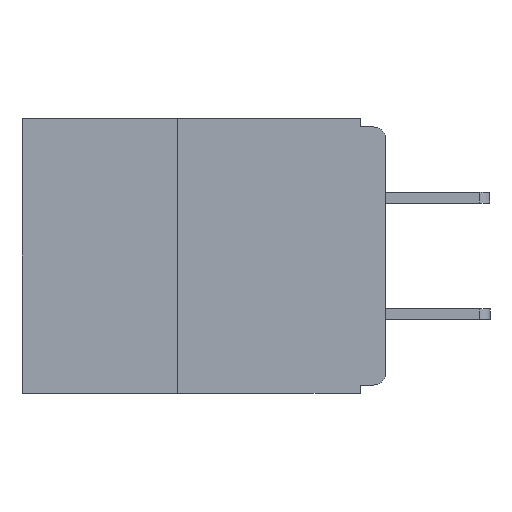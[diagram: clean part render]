
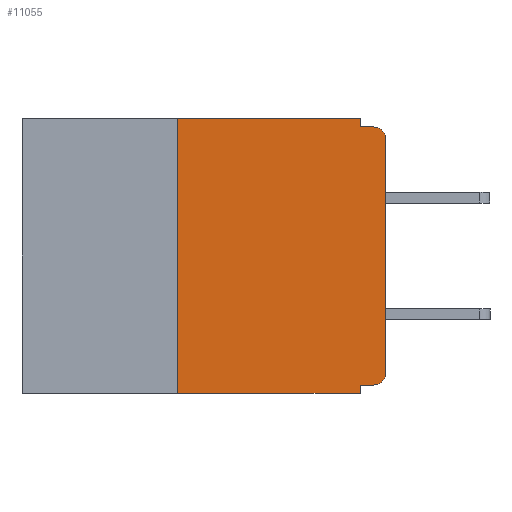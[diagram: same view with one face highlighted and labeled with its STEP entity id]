
A CAD part, left-side view. The second image highlights one B-rep face of the part: STEP entity #11055.
In plain terms, the highlighted planar face has unit normal (-1, 0, 0).
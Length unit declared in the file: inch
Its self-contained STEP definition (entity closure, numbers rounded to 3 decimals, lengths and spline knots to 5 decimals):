
#9 = VECTOR ( 'NONE', #11771, 39.37008 ) ;
#267 = DIRECTION ( 'NONE',  ( 0., 1., 0. ) ) ;
#414 = DIRECTION ( 'NONE',  ( 0., 0., -1. ) ) ;
#440 = ORIENTED_EDGE ( 'NONE', *, *, #5736, .T. ) ;
#484 = AXIS2_PLACEMENT_3D ( 'NONE', #6785, #6767, #6724 ) ;
#1037 = VECTOR ( 'NONE', #15498, 39.37008 ) ;
#1721 = EDGE_CURVE ( 'NONE', #16493, #3948, #3921, .T. ) ;
#1986 = FACE_OUTER_BOUND ( 'NONE', #13080, .T. ) ;
#2492 = EDGE_CURVE ( 'NONE', #4934, #12769, #3906, .T. ) ;
#2823 = LINE ( 'NONE', #11462, #10269 ) ;
#3153 = DIRECTION ( 'NONE',  ( 0., 0., 1. ) ) ;
#3399 = VERTEX_POINT ( 'NONE', #6399 ) ;
#3489 = CARTESIAN_POINT ( 'NONE',  ( 0., 0.031, 0. ) ) ;
#3809 = CARTESIAN_POINT ( 'NONE',  ( 0., 0., -0.32 ) ) ;
#3897 = CARTESIAN_POINT ( 'NONE',  ( 0., 0.031, -0.01 ) ) ;
#3906 = LINE ( 'NONE', #8156, #9 ) ;
#3921 = LINE ( 'NONE', #3809, #10933 ) ;
#3948 = VERTEX_POINT ( 'NONE', #5314 ) ;
#4382 = CARTESIAN_POINT ( 'NONE',  ( 0., 0., -0.305 ) ) ;
#4439 = CIRCLE ( 'NONE', #484, 0.015 ) ;
#4491 = DIRECTION ( 'NONE',  ( 0., -1., 0. ) ) ;
#4507 = CARTESIAN_POINT ( 'NONE',  ( 0., 0., -0.01 ) ) ;
#4882 = CARTESIAN_POINT ( 'NONE',  ( 0., 0.015, -0.01 ) ) ;
#4893 = VERTEX_POINT ( 'NONE', #4382 ) ;
#4934 = VERTEX_POINT ( 'NONE', #3489 ) ;
#5068 = LINE ( 'NONE', #12923, #12926 ) ;
#5070 = LINE ( 'NONE', #6970, #8335 ) ;
#5104 = VECTOR ( 'NONE', #5201, 39.37008 ) ;
#5185 = CARTESIAN_POINT ( 'NONE',  ( 0., 0.031, -0.33 ) ) ;
#5201 = DIRECTION ( 'NONE',  ( 0., 0., -1. ) ) ;
#5314 = CARTESIAN_POINT ( 'NONE',  ( 0., 0.031, -0.32 ) ) ;
#5357 = CARTESIAN_POINT ( 'NONE',  ( 0., 0.015, -0.32 ) ) ;
#5736 = EDGE_CURVE ( 'NONE', #4893, #9461, #15853, .T. ) ;
#5773 = ORIENTED_EDGE ( 'NONE', *, *, #7861, .F. ) ;
#6264 = VECTOR ( 'NONE', #4491, 39.37008 ) ;
#6399 = CARTESIAN_POINT ( 'NONE',  ( 0., 0.031, -0.33 ) ) ;
#6601 = ORIENTED_EDGE ( 'NONE', *, *, #16227, .T. ) ;
#6724 = DIRECTION ( 'NONE',  ( 0., 0., -1. ) ) ;
#6767 = DIRECTION ( 'NONE',  ( -1., 0., 0. ) ) ;
#6785 = CARTESIAN_POINT ( 'NONE',  ( 0., 0.015, -0.025 ) ) ;
#6944 = ORIENTED_EDGE ( 'NONE', *, *, #11170, .T. ) ;
#6970 = CARTESIAN_POINT ( 'NONE',  ( 0., 0.437, -0.33 ) ) ;
#7042 = ORIENTED_EDGE ( 'NONE', *, *, #12254, .T. ) ;
#7093 = ORIENTED_EDGE ( 'NONE', *, *, #14931, .F. ) ;
#7138 = LINE ( 'NONE', #4507, #6264 ) ;
#7443 = VERTEX_POINT ( 'NONE', #14865 ) ;
#7861 = EDGE_CURVE ( 'NONE', #7443, #4934, #2823, .T. ) ;
#7935 = DIRECTION ( 'NONE',  ( 0., 0., -1. ) ) ;
#7958 = DIRECTION ( 'NONE',  ( 1., 0., 0. ) ) ;
#8077 = CARTESIAN_POINT ( 'NONE',  ( 0., 0.437, 0. ) ) ;
#8149 = ORIENTED_EDGE ( 'NONE', *, *, #8701, .F. ) ;
#8156 = CARTESIAN_POINT ( 'NONE',  ( 0., 0.031, 0. ) ) ;
#8196 = PLANE ( 'NONE',  #12935 ) ;
#8335 = VECTOR ( 'NONE', #17702, 39.37008 ) ;
#8616 = VERTEX_POINT ( 'NONE', #4882 ) ;
#8701 = EDGE_CURVE ( 'NONE', #12769, #8616, #7138, .T. ) ;
#8972 = DIRECTION ( 'NONE',  ( -1., 0., 0. ) ) ;
#9232 = VERTEX_POINT ( 'NONE', #17607 ) ;
#9461 = VERTEX_POINT ( 'NONE', #12193 ) ;
#10269 = VECTOR ( 'NONE', #11386, 39.37008 ) ;
#10763 = AXIS2_PLACEMENT_3D ( 'NONE', #17027, #8972, #414 ) ;
#10933 = VECTOR ( 'NONE', #267, 39.37008 ) ;
#11055 = ADVANCED_FACE ( 'NONE', ( #1986 ), #8196, .F. ) ;
#11170 = EDGE_CURVE ( 'NONE', #9461, #8616, #4439, .T. ) ;
#11305 = EDGE_CURVE ( 'NONE', #3948, #3399, #12540, .T. ) ;
#11386 = DIRECTION ( 'NONE',  ( 0., -1., 0. ) ) ;
#11462 = CARTESIAN_POINT ( 'NONE',  ( 0., 0.437, 0. ) ) ;
#11667 = ORIENTED_EDGE ( 'NONE', *, *, #2492, .F. ) ;
#11771 = DIRECTION ( 'NONE',  ( 0., 0., -1. ) ) ;
#11865 = ORIENTED_EDGE ( 'NONE', *, *, #1721, .F. ) ;
#12193 = CARTESIAN_POINT ( 'NONE',  ( 0., 0., -0.025 ) ) ;
#12254 = EDGE_CURVE ( 'NONE', #9232, #3399, #5070, .T. ) ;
#12540 = LINE ( 'NONE', #5185, #5104 ) ;
#12769 = VERTEX_POINT ( 'NONE', #3897 ) ;
#12923 = CARTESIAN_POINT ( 'NONE',  ( 0., 0.25, -0.33 ) ) ;
#12926 = VECTOR ( 'NONE', #3153, 39.37008 ) ;
#12935 = AXIS2_PLACEMENT_3D ( 'NONE', #8077, #7958, #7935 ) ;
#13080 = EDGE_LOOP ( 'NONE', ( #440, #6944, #8149, #11667, #5773, #7093, #7042, #14428, #11865, #6601 ) ) ;
#14428 = ORIENTED_EDGE ( 'NONE', *, *, #11305, .F. ) ;
#14865 = CARTESIAN_POINT ( 'NONE',  ( 0., 0.25, 0. ) ) ;
#14931 = EDGE_CURVE ( 'NONE', #9232, #7443, #5068, .T. ) ;
#15498 = DIRECTION ( 'NONE',  ( 0., 0., 1. ) ) ;
#15560 = CIRCLE ( 'NONE', #10763, 0.015 ) ;
#15669 = CARTESIAN_POINT ( 'NONE',  ( 0., 0., 0. ) ) ;
#15853 = LINE ( 'NONE', #15669, #1037 ) ;
#16227 = EDGE_CURVE ( 'NONE', #16493, #4893, #15560, .T. ) ;
#16493 = VERTEX_POINT ( 'NONE', #5357 ) ;
#17027 = CARTESIAN_POINT ( 'NONE',  ( 0., 0.015, -0.305 ) ) ;
#17607 = CARTESIAN_POINT ( 'NONE',  ( 0., 0.25, -0.33 ) ) ;
#17702 = DIRECTION ( 'NONE',  ( 0., -1., 0. ) ) ;
